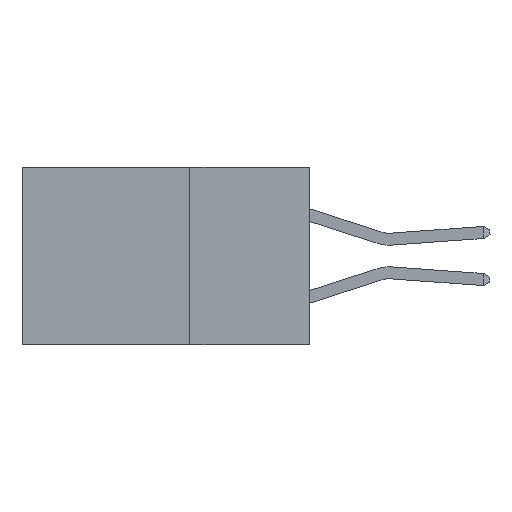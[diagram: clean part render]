
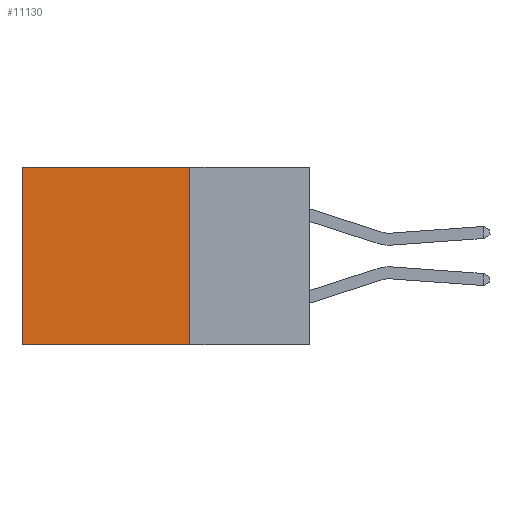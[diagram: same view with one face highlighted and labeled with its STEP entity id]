
A CAD part, left-side view. The second image highlights one B-rep face of the part: STEP entity #11130.
In plain terms, the highlighted planar face has unit normal (-1, 0, 0).
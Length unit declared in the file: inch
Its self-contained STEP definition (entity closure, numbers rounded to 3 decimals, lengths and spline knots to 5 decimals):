
#313 = VECTOR ( 'NONE', #1255, 39.37008 ) ;
#412 = ORIENTED_EDGE ( 'NONE', *, *, #9919, .T. ) ;
#500 = EDGE_LOOP ( 'NONE', ( #956, #13541, #10353, #412 ) ) ;
#856 = CARTESIAN_POINT ( 'NONE',  ( 0.298, 0.25, -0.37 ) ) ;
#956 = ORIENTED_EDGE ( 'NONE', *, *, #7325, .T. ) ;
#1255 = DIRECTION ( 'NONE',  ( 0., 1., 0. ) ) ;
#2376 = LINE ( 'NONE', #8304, #313 ) ;
#2893 = AXIS2_PLACEMENT_3D ( 'NONE', #11378, #12570, #5559 ) ;
#3601 = FACE_OUTER_BOUND ( 'NONE', #500, .T. ) ;
#3937 = EDGE_CURVE ( 'NONE', #13097, #6153, #7880, .T. ) ;
#5135 = VECTOR ( 'NONE', #9074, 39.37008 ) ;
#5190 = CARTESIAN_POINT ( 'NONE',  ( 0.298, 0.6, 0. ) ) ;
#5559 = DIRECTION ( 'NONE',  ( 0., 0., -1. ) ) ;
#6153 = VERTEX_POINT ( 'NONE', #11213 ) ;
#6477 = LINE ( 'NONE', #7158, #9195 ) ;
#7158 = CARTESIAN_POINT ( 'NONE',  ( 0.298, 0.6, 0. ) ) ;
#7325 = EDGE_CURVE ( 'NONE', #10143, #12409, #6477, .T. ) ;
#7880 = LINE ( 'NONE', #9088, #5135 ) ;
#7936 = LINE ( 'NONE', #856, #11029 ) ;
#8304 = CARTESIAN_POINT ( 'NONE',  ( 0.298, 0.25, 0. ) ) ;
#9015 = PLANE ( 'NONE',  #2893 ) ;
#9067 = DIRECTION ( 'NONE',  ( 0., 1., 0. ) ) ;
#9074 = DIRECTION ( 'NONE',  ( 0., 0., -1. ) ) ;
#9088 = CARTESIAN_POINT ( 'NONE',  ( 0.298, 0.25, 0. ) ) ;
#9195 = VECTOR ( 'NONE', #12991, 39.37008 ) ;
#9919 = EDGE_CURVE ( 'NONE', #13097, #10143, #2376, .T. ) ;
#10143 = VERTEX_POINT ( 'NONE', #5190 ) ;
#10353 = ORIENTED_EDGE ( 'NONE', *, *, #3937, .F. ) ;
#10454 = CARTESIAN_POINT ( 'NONE',  ( 0.298, 0.25, 0. ) ) ;
#11029 = VECTOR ( 'NONE', #9067, 39.37008 ) ;
#11130 = ADVANCED_FACE ( 'NONE', ( #3601 ), #9015, .F. ) ;
#11213 = CARTESIAN_POINT ( 'NONE',  ( 0.298, 0.25, -0.37 ) ) ;
#11378 = CARTESIAN_POINT ( 'NONE',  ( 0.298, 0.25, 0. ) ) ;
#12409 = VERTEX_POINT ( 'NONE', #13873 ) ;
#12570 = DIRECTION ( 'NONE',  ( 1., 0., 0. ) ) ;
#12916 = EDGE_CURVE ( 'NONE', #6153, #12409, #7936, .T. ) ;
#12991 = DIRECTION ( 'NONE',  ( 0., 0., -1. ) ) ;
#13097 = VERTEX_POINT ( 'NONE', #10454 ) ;
#13541 = ORIENTED_EDGE ( 'NONE', *, *, #12916, .F. ) ;
#13873 = CARTESIAN_POINT ( 'NONE',  ( 0.298, 0.6, -0.37 ) ) ;
